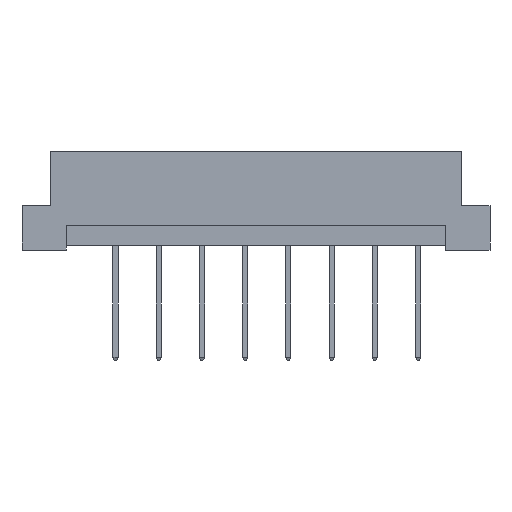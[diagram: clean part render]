
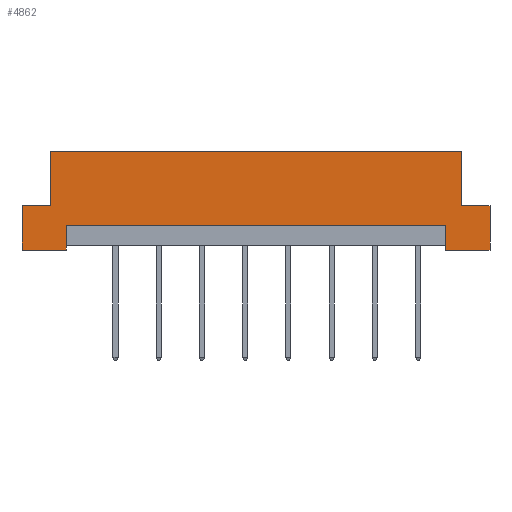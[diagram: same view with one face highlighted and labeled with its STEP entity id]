
A CAD part, front view. The second image highlights one B-rep face of the part: STEP entity #4862.
In plain terms, the highlighted planar face has unit normal (0, -1, 0).
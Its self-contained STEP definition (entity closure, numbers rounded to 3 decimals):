
#68 = DIRECTION ( 'NONE',  ( 0., 0., 1. ) ) ;
#158 = FACE_OUTER_BOUND ( 'NONE', #7548, .T. ) ;
#228 = VECTOR ( 'NONE', #2218, 1000. ) ;
#334 = CARTESIAN_POINT ( 'NONE',  ( -27.5, 0., 0. ) ) ;
#454 = EDGE_CURVE ( 'NONE', #2449, #4927, #5652, .T. ) ;
#718 = VERTEX_POINT ( 'NONE', #6794 ) ;
#783 = LINE ( 'NONE', #8478, #228 ) ;
#991 = VECTOR ( 'NONE', #2732, 1000. ) ;
#1003 = CARTESIAN_POINT ( 'NONE',  ( -27.5, 0., 5.2 ) ) ;
#1139 = ORIENTED_EDGE ( 'NONE', *, *, #2006, .F. ) ;
#1345 = EDGE_CURVE ( 'NONE', #4927, #4985, #8005, .T. ) ;
#1354 = VECTOR ( 'NONE', #6683, 1000. ) ;
#1436 = LINE ( 'NONE', #1485, #8850 ) ;
#1485 = CARTESIAN_POINT ( 'NONE',  ( -24.2, 0., 5.2 ) ) ;
#1499 = ORIENTED_EDGE ( 'NONE', *, *, #7906, .F. ) ;
#1589 = ORIENTED_EDGE ( 'NONE', *, *, #4198, .F. ) ;
#1660 = DIRECTION ( 'NONE',  ( 0., 0., -1. ) ) ;
#1757 = CARTESIAN_POINT ( 'NONE',  ( -27.5, 0., 0. ) ) ;
#1867 = LINE ( 'NONE', #1003, #2844 ) ;
#2006 = EDGE_CURVE ( 'NONE', #4985, #6599, #5903, .T. ) ;
#2104 = CARTESIAN_POINT ( 'NONE',  ( 22.3, 0., 2.9 ) ) ;
#2170 = CARTESIAN_POINT ( 'NONE',  ( -27.5, 0., 0. ) ) ;
#2218 = DIRECTION ( 'NONE',  ( 1., 0., 0. ) ) ;
#2219 = EDGE_CURVE ( 'NONE', #7365, #6599, #4030, .T. ) ;
#2321 = EDGE_CURVE ( 'NONE', #5830, #6580, #7042, .T. ) ;
#2415 = ORIENTED_EDGE ( 'NONE', *, *, #5902, .T. ) ;
#2449 = VERTEX_POINT ( 'NONE', #4570 ) ;
#2558 = LINE ( 'NONE', #4103, #8405 ) ;
#2732 = DIRECTION ( 'NONE',  ( 0., 0., -1. ) ) ;
#2844 = VECTOR ( 'NONE', #4512, 1000. ) ;
#2898 = DIRECTION ( 'NONE',  ( 0., 0., 1. ) ) ;
#2956 = PLANE ( 'NONE',  #7428 ) ;
#3024 = CARTESIAN_POINT ( 'NONE',  ( 27.5, 0., 0. ) ) ;
#3030 = EDGE_CURVE ( 'NONE', #7035, #5939, #3416, .T. ) ;
#3187 = ORIENTED_EDGE ( 'NONE', *, *, #2321, .F. ) ;
#3333 = DIRECTION ( 'NONE',  ( -1., 0., 0. ) ) ;
#3416 = LINE ( 'NONE', #9013, #991 ) ;
#3437 = DIRECTION ( 'NONE',  ( 0., 0., -1. ) ) ;
#3470 = LINE ( 'NONE', #2104, #8307 ) ;
#3561 = CARTESIAN_POINT ( 'NONE',  ( -27.5, 0., 5.2 ) ) ;
#4030 = LINE ( 'NONE', #6273, #6015 ) ;
#4085 = VECTOR ( 'NONE', #8243, 1000. ) ;
#4103 = CARTESIAN_POINT ( 'NONE',  ( -27.5, 0., 0. ) ) ;
#4198 = EDGE_CURVE ( 'NONE', #5939, #5830, #2558, .T. ) ;
#4512 = DIRECTION ( 'NONE',  ( 1., 0., 0. ) ) ;
#4570 = CARTESIAN_POINT ( 'NONE',  ( 24.2, 0., 5.2 ) ) ;
#4632 = CARTESIAN_POINT ( 'NONE',  ( -22.3, 0., 0. ) ) ;
#4767 = CARTESIAN_POINT ( 'NONE',  ( -24.2, 0., 5.2 ) ) ;
#4788 = DIRECTION ( 'NONE',  ( 1., 0., 0. ) ) ;
#4862 = ADVANCED_FACE ( 'NONE', ( #158 ), #2956, .F. ) ;
#4927 = VERTEX_POINT ( 'NONE', #5210 ) ;
#4985 = VERTEX_POINT ( 'NONE', #5862 ) ;
#4998 = ORIENTED_EDGE ( 'NONE', *, *, #3030, .F. ) ;
#4999 = CARTESIAN_POINT ( 'NONE',  ( 22.3, 0., 2.9 ) ) ;
#5210 = CARTESIAN_POINT ( 'NONE',  ( 27.5, 0., 5.2 ) ) ;
#5552 = CARTESIAN_POINT ( 'NONE',  ( 27.5, 0., 5.2 ) ) ;
#5557 = VERTEX_POINT ( 'NONE', #6801 ) ;
#5599 = DIRECTION ( 'NONE',  ( -1., 0., 0. ) ) ;
#5652 = LINE ( 'NONE', #5552, #8020 ) ;
#5685 = CARTESIAN_POINT ( 'NONE',  ( -22.3, 0., 2.9 ) ) ;
#5726 = CARTESIAN_POINT ( 'NONE',  ( -27.5, 0., 11.6 ) ) ;
#5830 = VERTEX_POINT ( 'NONE', #334 ) ;
#5862 = CARTESIAN_POINT ( 'NONE',  ( 27.5, 0., 0. ) ) ;
#5902 = EDGE_CURVE ( 'NONE', #2449, #718, #8158, .T. ) ;
#5903 = LINE ( 'NONE', #1757, #1354 ) ;
#5905 = ORIENTED_EDGE ( 'NONE', *, *, #6600, .F. ) ;
#5939 = VERTEX_POINT ( 'NONE', #4632 ) ;
#6015 = VECTOR ( 'NONE', #3437, 1000. ) ;
#6164 = VECTOR ( 'NONE', #2898, 1000. ) ;
#6273 = CARTESIAN_POINT ( 'NONE',  ( 22.3, 0., 0.5 ) ) ;
#6363 = DIRECTION ( 'NONE',  ( 0., 0., 1. ) ) ;
#6469 = EDGE_CURVE ( 'NONE', #7365, #7035, #3470, .T. ) ;
#6580 = VERTEX_POINT ( 'NONE', #3561 ) ;
#6599 = VERTEX_POINT ( 'NONE', #8037 ) ;
#6600 = EDGE_CURVE ( 'NONE', #6580, #7270, #1867, .T. ) ;
#6683 = DIRECTION ( 'NONE',  ( -1., 0., 0. ) ) ;
#6753 = VECTOR ( 'NONE', #1660, 1000. ) ;
#6794 = CARTESIAN_POINT ( 'NONE',  ( 24.2, 0., 11.6 ) ) ;
#6801 = CARTESIAN_POINT ( 'NONE',  ( -24.2, 0., 11.6 ) ) ;
#6865 = ORIENTED_EDGE ( 'NONE', *, *, #454, .F. ) ;
#6918 = ORIENTED_EDGE ( 'NONE', *, *, #2219, .T. ) ;
#7011 = DIRECTION ( 'NONE',  ( 0., 1., 0. ) ) ;
#7035 = VERTEX_POINT ( 'NONE', #5685 ) ;
#7042 = LINE ( 'NONE', #2170, #6164 ) ;
#7127 = ORIENTED_EDGE ( 'NONE', *, *, #1345, .F. ) ;
#7270 = VERTEX_POINT ( 'NONE', #4767 ) ;
#7365 = VERTEX_POINT ( 'NONE', #4999 ) ;
#7428 = AXIS2_PLACEMENT_3D ( 'NONE', #5726, #7011, #68 ) ;
#7548 = EDGE_LOOP ( 'NONE', ( #8940, #6918, #1139, #7127, #6865, #2415, #1499, #7834, #5905, #3187, #1589, #4998 ) ) ;
#7818 = EDGE_CURVE ( 'NONE', #7270, #5557, #1436, .T. ) ;
#7834 = ORIENTED_EDGE ( 'NONE', *, *, #7818, .F. ) ;
#7906 = EDGE_CURVE ( 'NONE', #5557, #718, #783, .T. ) ;
#8005 = LINE ( 'NONE', #3024, #6753 ) ;
#8020 = VECTOR ( 'NONE', #4788, 1000. ) ;
#8037 = CARTESIAN_POINT ( 'NONE',  ( 22.3, 0., 0. ) ) ;
#8158 = LINE ( 'NONE', #8204, #4085 ) ;
#8204 = CARTESIAN_POINT ( 'NONE',  ( 24.2, 0., 5.2 ) ) ;
#8243 = DIRECTION ( 'NONE',  ( 0., 0., 1. ) ) ;
#8307 = VECTOR ( 'NONE', #5599, 1000. ) ;
#8405 = VECTOR ( 'NONE', #3333, 1000. ) ;
#8478 = CARTESIAN_POINT ( 'NONE',  ( -27.5, 0., 11.6 ) ) ;
#8850 = VECTOR ( 'NONE', #6363, 1000. ) ;
#8940 = ORIENTED_EDGE ( 'NONE', *, *, #6469, .F. ) ;
#9013 = CARTESIAN_POINT ( 'NONE',  ( -22.3, 0., 0.5 ) ) ;
